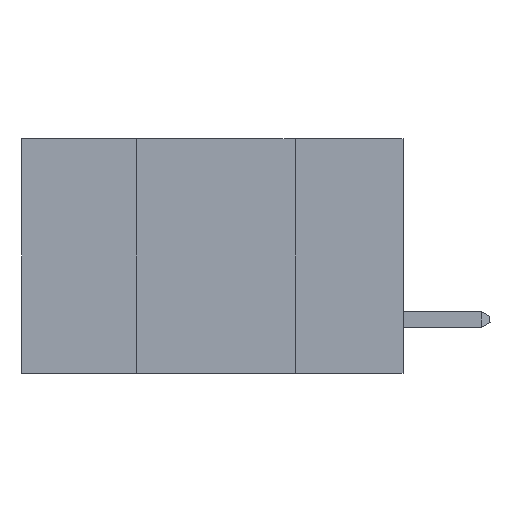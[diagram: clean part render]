
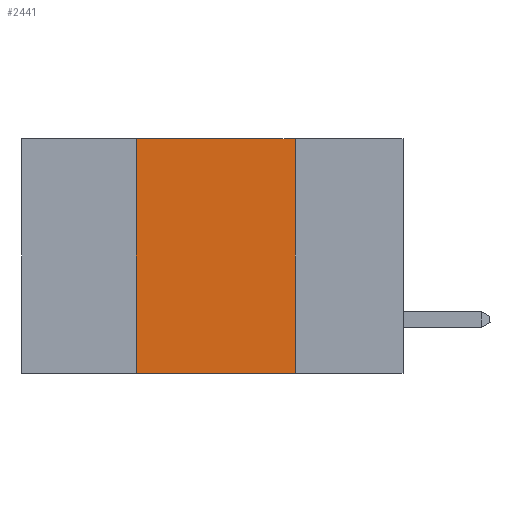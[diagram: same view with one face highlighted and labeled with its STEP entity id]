
A CAD part, left-side view. The second image highlights one B-rep face of the part: STEP entity #2441.
In plain terms, the highlighted planar face has unit normal (-1, 0, 0).
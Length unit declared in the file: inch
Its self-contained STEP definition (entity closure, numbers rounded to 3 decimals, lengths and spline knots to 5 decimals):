
#63 = EDGE_CURVE ( 'NONE', #17714, #11382, #20273, .T. ) ;
#382 = EDGE_CURVE ( 'NONE', #8000, #21026, #16912, .T. ) ;
#684 = VECTOR ( 'NONE', #10095, 39.37008 ) ;
#1078 = EDGE_LOOP ( 'NONE', ( #17795, #9291, #12811, #16393 ) ) ;
#1362 = CARTESIAN_POINT ( 'NONE',  ( 0., 0.42, -0.37 ) ) ;
#1554 = VECTOR ( 'NONE', #12976, 39.37008 ) ;
#2032 = CARTESIAN_POINT ( 'NONE',  ( 0., 0.17, -0.37 ) ) ;
#2441 = ADVANCED_FACE ( 'NONE', ( #2735 ), #8664, .F. ) ;
#2735 = FACE_OUTER_BOUND ( 'NONE', #1078, .T. ) ;
#2831 = EDGE_CURVE ( 'NONE', #11382, #8000, #10477, .T. ) ;
#3898 = VECTOR ( 'NONE', #7796, 39.37008 ) ;
#4488 = CARTESIAN_POINT ( 'NONE',  ( 0., 0.42, 0. ) ) ;
#5562 = DIRECTION ( 'NONE',  ( 1., 0., 0. ) ) ;
#6575 = AXIS2_PLACEMENT_3D ( 'NONE', #13608, #5562, #20297 ) ;
#7120 = CARTESIAN_POINT ( 'NONE',  ( 0., 0.6, -0.37 ) ) ;
#7796 = DIRECTION ( 'NONE',  ( 0., 0., 1. ) ) ;
#8000 = VERTEX_POINT ( 'NONE', #17300 ) ;
#8664 = PLANE ( 'NONE',  #6575 ) ;
#8925 = DIRECTION ( 'NONE',  ( 0., -1., 0. ) ) ;
#9023 = CARTESIAN_POINT ( 'NONE',  ( 0., 0.42, 0. ) ) ;
#9291 = ORIENTED_EDGE ( 'NONE', *, *, #2831, .F. ) ;
#9784 = VECTOR ( 'NONE', #8925, 39.37008 ) ;
#10095 = DIRECTION ( 'NONE',  ( 0., -1., 0. ) ) ;
#10477 = LINE ( 'NONE', #18300, #684 ) ;
#11382 = VERTEX_POINT ( 'NONE', #9023 ) ;
#11833 = EDGE_CURVE ( 'NONE', #17714, #21026, #14346, .T. ) ;
#12811 = ORIENTED_EDGE ( 'NONE', *, *, #63, .F. ) ;
#12976 = DIRECTION ( 'NONE',  ( 0., 0., -1. ) ) ;
#13608 = CARTESIAN_POINT ( 'NONE',  ( 0., 0.6, 0. ) ) ;
#14346 = LINE ( 'NONE', #7120, #9784 ) ;
#16393 = ORIENTED_EDGE ( 'NONE', *, *, #11833, .T. ) ;
#16912 = LINE ( 'NONE', #19579, #1554 ) ;
#17300 = CARTESIAN_POINT ( 'NONE',  ( 0., 0.17, 0. ) ) ;
#17714 = VERTEX_POINT ( 'NONE', #1362 ) ;
#17795 = ORIENTED_EDGE ( 'NONE', *, *, #382, .F. ) ;
#18300 = CARTESIAN_POINT ( 'NONE',  ( 0., 0.6, 0. ) ) ;
#19579 = CARTESIAN_POINT ( 'NONE',  ( 0., 0.17, 0. ) ) ;
#20273 = LINE ( 'NONE', #4488, #3898 ) ;
#20297 = DIRECTION ( 'NONE',  ( 0., 0., -1. ) ) ;
#21026 = VERTEX_POINT ( 'NONE', #2032 ) ;
